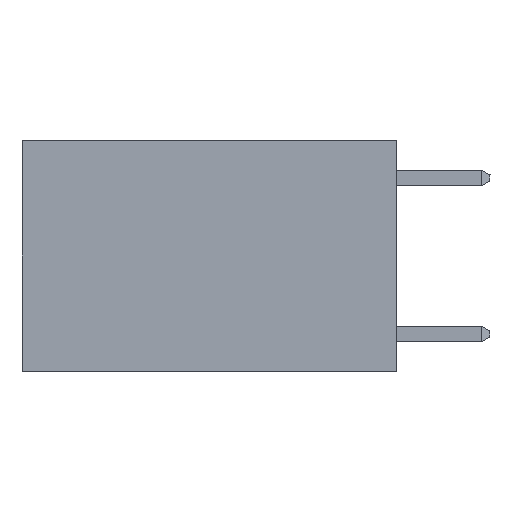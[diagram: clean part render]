
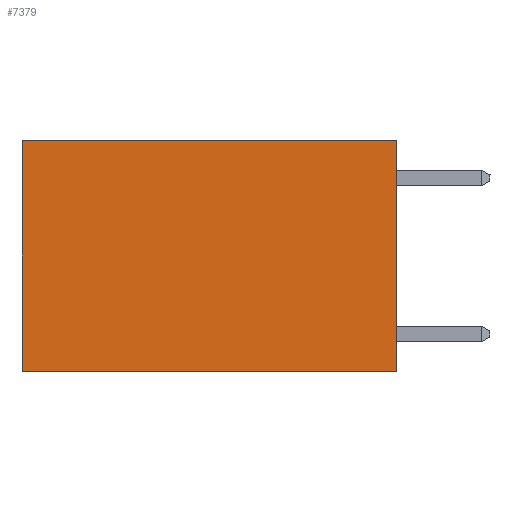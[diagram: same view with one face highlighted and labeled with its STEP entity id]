
A CAD part, left-side view. The second image highlights one B-rep face of the part: STEP entity #7379.
In plain terms, the highlighted planar face has unit normal (-1, 0, 0).
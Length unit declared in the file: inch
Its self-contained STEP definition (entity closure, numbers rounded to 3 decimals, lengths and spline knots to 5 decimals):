
#83 = VERTEX_POINT ( 'NONE', #5100 ) ;
#333 = ORIENTED_EDGE ( 'NONE', *, *, #2707, .F. ) ;
#639 = DIRECTION ( 'NONE',  ( 0., 0., -1. ) ) ;
#776 = LINE ( 'NONE', #1539, #6020 ) ;
#888 = VERTEX_POINT ( 'NONE', #4144 ) ;
#953 = EDGE_CURVE ( 'NONE', #83, #888, #4267, .T. ) ;
#972 = LINE ( 'NONE', #3490, #1351 ) ;
#1062 = ORIENTED_EDGE ( 'NONE', *, *, #5685, .F. ) ;
#1351 = VECTOR ( 'NONE', #3933, 39.37008 ) ;
#1539 = CARTESIAN_POINT ( 'NONE',  ( 0.2625, 0., 0. ) ) ;
#1804 = VECTOR ( 'NONE', #639, 39.37008 ) ;
#1834 = CARTESIAN_POINT ( 'NONE',  ( 0.2625, 0.6, 0. ) ) ;
#2374 = CARTESIAN_POINT ( 'NONE',  ( 0.2625, 0., 0. ) ) ;
#2473 = EDGE_CURVE ( 'NONE', #3016, #83, #776, .T. ) ;
#2707 = EDGE_CURVE ( 'NONE', #5107, #888, #972, .T. ) ;
#2988 = PLANE ( 'NONE',  #6039 ) ;
#3016 = VERTEX_POINT ( 'NONE', #5934 ) ;
#3490 = CARTESIAN_POINT ( 'NONE',  ( 0.2625, 0., -0.37 ) ) ;
#3556 = EDGE_LOOP ( 'NONE', ( #4928, #333, #1062, #7121 ) ) ;
#3933 = DIRECTION ( 'NONE',  ( 0., 1., 0. ) ) ;
#4144 = CARTESIAN_POINT ( 'NONE',  ( 0.2625, 0.6, -0.37 ) ) ;
#4267 = LINE ( 'NONE', #1834, #1804 ) ;
#4889 = CARTESIAN_POINT ( 'NONE',  ( 0.2625, 0., 0. ) ) ;
#4928 = ORIENTED_EDGE ( 'NONE', *, *, #953, .T. ) ;
#5100 = CARTESIAN_POINT ( 'NONE',  ( 0.2625, 0.6, 0. ) ) ;
#5107 = VERTEX_POINT ( 'NONE', #5335 ) ;
#5335 = CARTESIAN_POINT ( 'NONE',  ( 0.2625, 0., -0.37 ) ) ;
#5547 = LINE ( 'NONE', #2374, #6792 ) ;
#5685 = EDGE_CURVE ( 'NONE', #3016, #5107, #5547, .T. ) ;
#5934 = CARTESIAN_POINT ( 'NONE',  ( 0.2625, 0., 0. ) ) ;
#6020 = VECTOR ( 'NONE', #7146, 39.37008 ) ;
#6039 = AXIS2_PLACEMENT_3D ( 'NONE', #4889, #6646, #6806 ) ;
#6041 = DIRECTION ( 'NONE',  ( 0., 0., -1. ) ) ;
#6646 = DIRECTION ( 'NONE',  ( 1., 0., 0. ) ) ;
#6689 = FACE_OUTER_BOUND ( 'NONE', #3556, .T. ) ;
#6792 = VECTOR ( 'NONE', #6041, 39.37008 ) ;
#6806 = DIRECTION ( 'NONE',  ( 0., 0., -1. ) ) ;
#7121 = ORIENTED_EDGE ( 'NONE', *, *, #2473, .T. ) ;
#7146 = DIRECTION ( 'NONE',  ( 0., 1., 0. ) ) ;
#7379 = ADVANCED_FACE ( 'NONE', ( #6689 ), #2988, .F. ) ;
